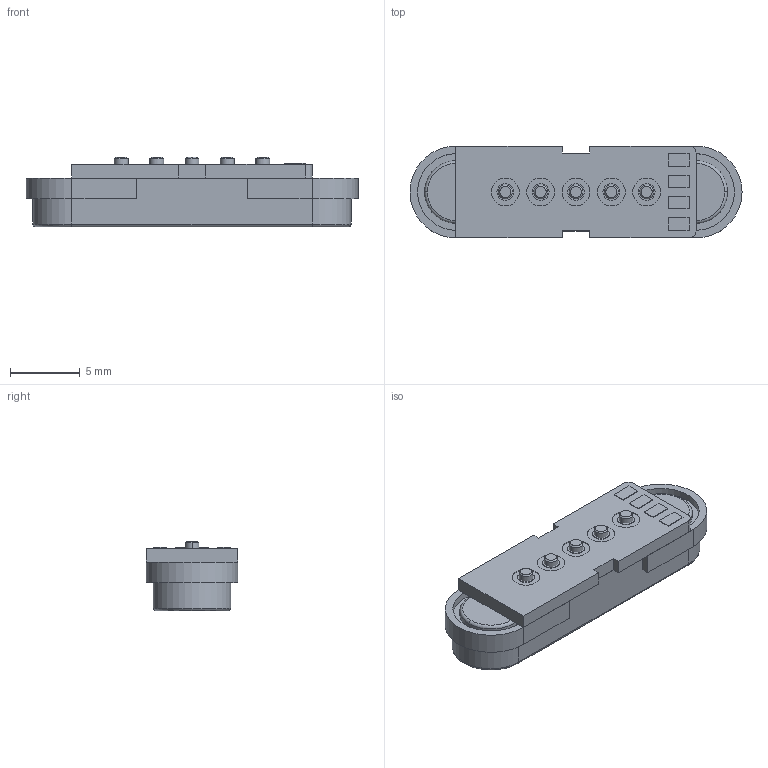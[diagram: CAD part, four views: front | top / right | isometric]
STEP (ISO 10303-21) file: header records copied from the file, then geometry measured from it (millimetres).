
FILE_DESCRIPTION (( 'STEP AP214' ), '1' );
FILE_NAME ('686D05C2P50110E.STEP', '2023-04-14T20:25:39', ( '' ), ( '' ), 'SwSTEP 2.0', 'SolidWorks 2020', '' );
FILE_SCHEMA (( 'AUTOMOTIVE_DESIGN' ));
Length unit declared in the file: millimetre
Products named in the file (1): 686D05C2P50110E
Bounding box: 23.86 x 6.6 x 5 mm (x, y, z)
Volume: 525.8 mm3; surface area: 930.2 mm2
Topology: 6 solids, 6 shells, 227 faces, 547 edges, 351 vertices
Faces by surface type: plane 102, cylinder 85, cone 20, bspline 14, torus 6
Entity records: 9879 total; most frequent: CARTESIAN_POINT 1998, DIRECTION 1129, ORIENTED_EDGE 1058, EDGE_CURVE 529, AXIS2_PLACEMENT_3D 414, VERTEX_POINT 347, LINE 301, VECTOR 301
